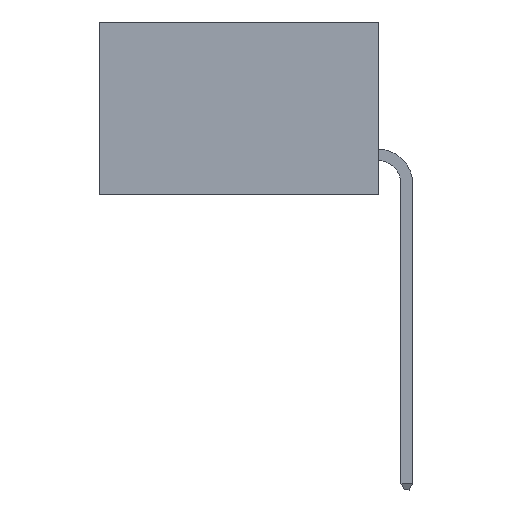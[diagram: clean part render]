
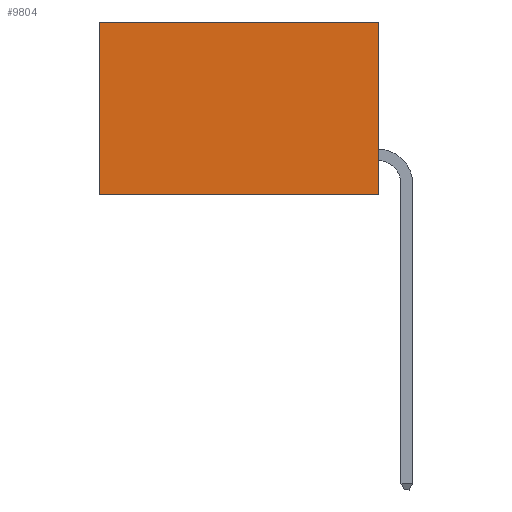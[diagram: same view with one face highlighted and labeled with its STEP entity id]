
A CAD part, left-side view. The second image highlights one B-rep face of the part: STEP entity #9804.
In plain terms, the highlighted planar face has unit normal (-1, 0, 0).
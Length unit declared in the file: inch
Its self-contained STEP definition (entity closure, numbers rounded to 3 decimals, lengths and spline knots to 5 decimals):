
#218 = VECTOR ( 'NONE', #8486, 39.37008 ) ;
#408 = LINE ( 'NONE', #11520, #3117 ) ;
#705 = CARTESIAN_POINT ( 'NONE',  ( 0.2615, 0., -0.37 ) ) ;
#1502 = VERTEX_POINT ( 'NONE', #8451 ) ;
#1519 = VERTEX_POINT ( 'NONE', #7430 ) ;
#2232 = LINE ( 'NONE', #3066, #5278 ) ;
#2443 = AXIS2_PLACEMENT_3D ( 'NONE', #3719, #6456, #10342 ) ;
#2745 = DIRECTION ( 'NONE',  ( 0., 1., 0. ) ) ;
#3066 = CARTESIAN_POINT ( 'NONE',  ( 0.2615, 0.6, -0.37 ) ) ;
#3117 = VECTOR ( 'NONE', #7019, 39.37008 ) ;
#3566 = EDGE_CURVE ( 'NONE', #1502, #11389, #408, .T. ) ;
#3719 = CARTESIAN_POINT ( 'NONE',  ( 0.2615, 0., -0.37 ) ) ;
#4329 = VECTOR ( 'NONE', #2745, 39.37008 ) ;
#4377 = EDGE_CURVE ( 'NONE', #1502, #5082, #7771, .T. ) ;
#5082 = VERTEX_POINT ( 'NONE', #705 ) ;
#5278 = VECTOR ( 'NONE', #7753, 39.37008 ) ;
#5379 = EDGE_CURVE ( 'NONE', #11389, #1519, #2232, .T. ) ;
#5608 = PLANE ( 'NONE',  #2443 ) ;
#5962 = EDGE_CURVE ( 'NONE', #5082, #1519, #8140, .T. ) ;
#6328 = CARTESIAN_POINT ( 'NONE',  ( 0.2615, 0.6, 0. ) ) ;
#6456 = DIRECTION ( 'NONE',  ( 1., 0., 0. ) ) ;
#7019 = DIRECTION ( 'NONE',  ( 0., 1., 0. ) ) ;
#7083 = ORIENTED_EDGE ( 'NONE', *, *, #3566, .T. ) ;
#7430 = CARTESIAN_POINT ( 'NONE',  ( 0.2615, 0.6, -0.37 ) ) ;
#7753 = DIRECTION ( 'NONE',  ( 0., 0., -1. ) ) ;
#7771 = LINE ( 'NONE', #9413, #218 ) ;
#8140 = LINE ( 'NONE', #9911, #4329 ) ;
#8443 = ORIENTED_EDGE ( 'NONE', *, *, #4377, .F. ) ;
#8451 = CARTESIAN_POINT ( 'NONE',  ( 0.2615, 0., 0. ) ) ;
#8486 = DIRECTION ( 'NONE',  ( 0., 0., -1. ) ) ;
#9372 = FACE_OUTER_BOUND ( 'NONE', #10484, .T. ) ;
#9413 = CARTESIAN_POINT ( 'NONE',  ( 0.2615, 0., -0.37 ) ) ;
#9804 = ADVANCED_FACE ( 'NONE', ( #9372 ), #5608, .F. ) ;
#9911 = CARTESIAN_POINT ( 'NONE',  ( 0.2615, 0., -0.37 ) ) ;
#10342 = DIRECTION ( 'NONE',  ( 0., 0., -1. ) ) ;
#10484 = EDGE_LOOP ( 'NONE', ( #10823, #11210, #8443, #7083 ) ) ;
#10823 = ORIENTED_EDGE ( 'NONE', *, *, #5379, .T. ) ;
#11210 = ORIENTED_EDGE ( 'NONE', *, *, #5962, .F. ) ;
#11389 = VERTEX_POINT ( 'NONE', #6328 ) ;
#11520 = CARTESIAN_POINT ( 'NONE',  ( 0.2615, 0., 0. ) ) ;
